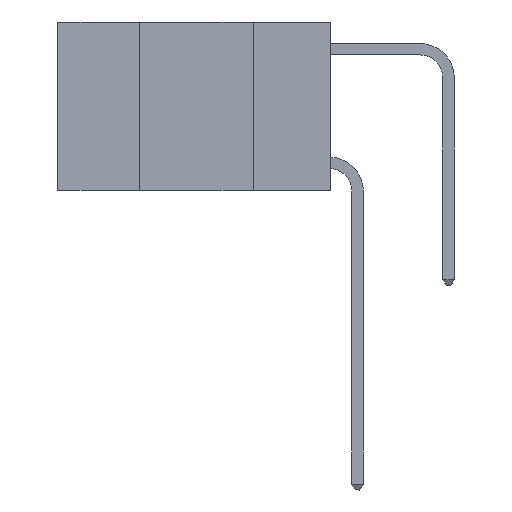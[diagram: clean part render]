
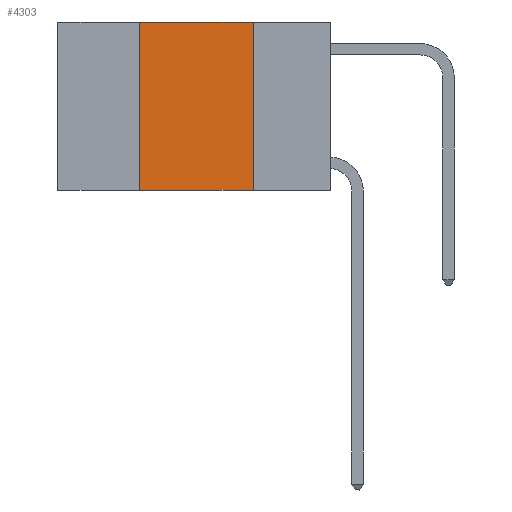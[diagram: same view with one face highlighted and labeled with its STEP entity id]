
A CAD part, left-side view. The second image highlights one B-rep face of the part: STEP entity #4303.
In plain terms, the highlighted planar face has unit normal (-1, 0, 0).
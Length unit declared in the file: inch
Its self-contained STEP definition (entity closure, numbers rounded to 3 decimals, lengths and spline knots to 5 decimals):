
#476 = CARTESIAN_POINT ( 'NONE',  ( 0., 0.42, -0.37 ) ) ;
#701 = LINE ( 'NONE', #2495, #6091 ) ;
#831 = DIRECTION ( 'NONE',  ( 0., -1., 0. ) ) ;
#1155 = EDGE_CURVE ( 'NONE', #4410, #5894, #10224, .T. ) ;
#2495 = CARTESIAN_POINT ( 'NONE',  ( 0., 0.42, 0. ) ) ;
#2538 = ORIENTED_EDGE ( 'NONE', *, *, #7610, .F. ) ;
#2597 = ORIENTED_EDGE ( 'NONE', *, *, #11904, .F. ) ;
#3106 = EDGE_LOOP ( 'NONE', ( #2538, #8126, #2597, #3151 ) ) ;
#3151 = ORIENTED_EDGE ( 'NONE', *, *, #10504, .T. ) ;
#4303 = ADVANCED_FACE ( 'NONE', ( #7980 ), #4862, .F. ) ;
#4410 = VERTEX_POINT ( 'NONE', #8148 ) ;
#4467 = VECTOR ( 'NONE', #831, 39.37008 ) ;
#4715 = VECTOR ( 'NONE', #11165, 39.37008 ) ;
#4862 = PLANE ( 'NONE',  #11299 ) ;
#5894 = VERTEX_POINT ( 'NONE', #7382 ) ;
#5922 = DIRECTION ( 'NONE',  ( 1., 0., 0. ) ) ;
#6091 = VECTOR ( 'NONE', #7667, 39.37008 ) ;
#7012 = VECTOR ( 'NONE', #8445, 39.37008 ) ;
#7233 = LINE ( 'NONE', #9606, #4467 ) ;
#7382 = CARTESIAN_POINT ( 'NONE',  ( 0., 0.17, 0. ) ) ;
#7442 = LINE ( 'NONE', #9465, #4715 ) ;
#7492 = CARTESIAN_POINT ( 'NONE',  ( 0., 0.17, -0.37 ) ) ;
#7610 = EDGE_CURVE ( 'NONE', #5894, #11771, #7442, .T. ) ;
#7667 = DIRECTION ( 'NONE',  ( 0., 0., 1. ) ) ;
#7980 = FACE_OUTER_BOUND ( 'NONE', #3106, .T. ) ;
#8126 = ORIENTED_EDGE ( 'NONE', *, *, #1155, .F. ) ;
#8148 = CARTESIAN_POINT ( 'NONE',  ( 0., 0.42, 0. ) ) ;
#8152 = CARTESIAN_POINT ( 'NONE',  ( 0., 0.6, 0. ) ) ;
#8445 = DIRECTION ( 'NONE',  ( 0., -1., 0. ) ) ;
#9465 = CARTESIAN_POINT ( 'NONE',  ( 0., 0.17, 0. ) ) ;
#9606 = CARTESIAN_POINT ( 'NONE',  ( 0., 0.6, -0.37 ) ) ;
#10197 = VERTEX_POINT ( 'NONE', #476 ) ;
#10224 = LINE ( 'NONE', #8152, #7012 ) ;
#10497 = CARTESIAN_POINT ( 'NONE',  ( 0., 0.6, 0. ) ) ;
#10504 = EDGE_CURVE ( 'NONE', #10197, #11771, #7233, .T. ) ;
#11165 = DIRECTION ( 'NONE',  ( 0., 0., -1. ) ) ;
#11299 = AXIS2_PLACEMENT_3D ( 'NONE', #10497, #5922, #12202 ) ;
#11771 = VERTEX_POINT ( 'NONE', #7492 ) ;
#11904 = EDGE_CURVE ( 'NONE', #10197, #4410, #701, .T. ) ;
#12202 = DIRECTION ( 'NONE',  ( 0., 0., -1. ) ) ;
